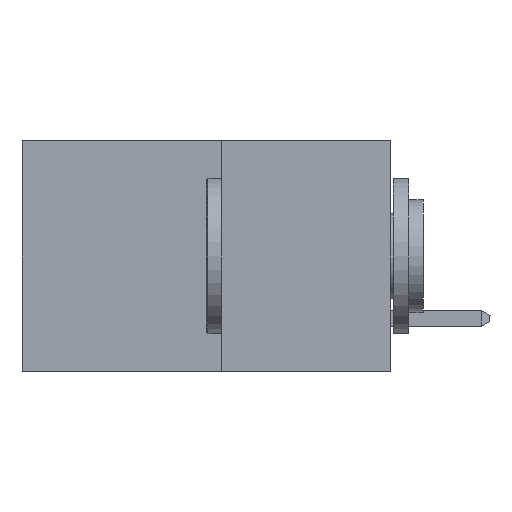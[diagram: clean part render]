
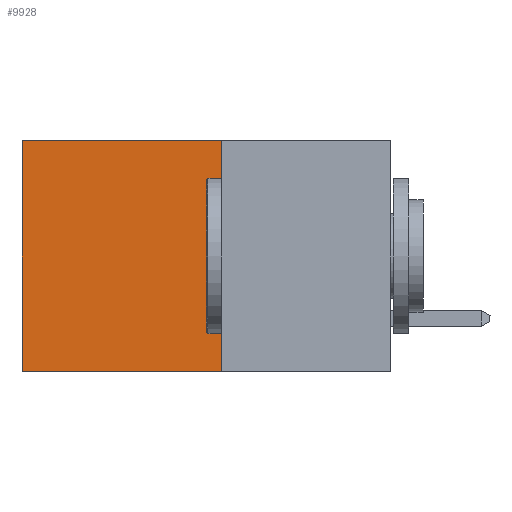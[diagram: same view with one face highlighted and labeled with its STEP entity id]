
A CAD part, left-side view. The second image highlights one B-rep face of the part: STEP entity #9928.
In plain terms, the highlighted planar face has unit normal (-1, 0, 0).
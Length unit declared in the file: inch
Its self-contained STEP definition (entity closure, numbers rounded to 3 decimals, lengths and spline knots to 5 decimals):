
#417 = DIRECTION ( 'NONE',  ( 0., 0., -1. ) ) ;
#490 = VECTOR ( 'NONE', #26340, 39.37008 ) ;
#1236 = ORIENTED_EDGE ( 'NONE', *, *, #13361, .F. ) ;
#3910 = CARTESIAN_POINT ( 'NONE',  ( 0.277, 0.59, 0. ) ) ;
#5032 = CARTESIAN_POINT ( 'NONE',  ( 0.277, 0.27, 0. ) ) ;
#5925 = LINE ( 'NONE', #8817, #16747 ) ;
#6266 = VERTEX_POINT ( 'NONE', #3910 ) ;
#6485 = VECTOR ( 'NONE', #9654, 39.37008 ) ;
#8775 = ORIENTED_EDGE ( 'NONE', *, *, #8777, .F. ) ;
#8777 = EDGE_CURVE ( 'NONE', #9025, #25424, #19285, .T. ) ;
#8817 = CARTESIAN_POINT ( 'NONE',  ( 0.277, 0.27, -0.37 ) ) ;
#9025 = VERTEX_POINT ( 'NONE', #25426 ) ;
#9540 = VERTEX_POINT ( 'NONE', #16863 ) ;
#9654 = DIRECTION ( 'NONE',  ( 0., 0., -1. ) ) ;
#9928 = ADVANCED_FACE ( 'NONE', ( #11229 ), #24043, .F. ) ;
#9935 = ORIENTED_EDGE ( 'NONE', *, *, #23583, .T. ) ;
#11036 = DIRECTION ( 'NONE',  ( 0., 1., 0. ) ) ;
#11229 = FACE_OUTER_BOUND ( 'NONE', #14681, .T. ) ;
#11257 = CARTESIAN_POINT ( 'NONE',  ( 0.277, 0.27, -0.37 ) ) ;
#11324 = EDGE_CURVE ( 'NONE', #6266, #9540, #26089, .T. ) ;
#11795 = CARTESIAN_POINT ( 'NONE',  ( 0.277, 0.27, -0.37 ) ) ;
#13361 = EDGE_CURVE ( 'NONE', #25424, #9540, #5925, .T. ) ;
#13459 = DIRECTION ( 'NONE',  ( 1., 0., 0. ) ) ;
#13855 = CARTESIAN_POINT ( 'NONE',  ( 0.277, 0.59, -0.37 ) ) ;
#14681 = EDGE_LOOP ( 'NONE', ( #19759, #1236, #8775, #9935 ) ) ;
#15970 = DIRECTION ( 'NONE',  ( 0., 0., -1. ) ) ;
#16747 = VECTOR ( 'NONE', #11036, 39.37008 ) ;
#16863 = CARTESIAN_POINT ( 'NONE',  ( 0.277, 0.59, -0.37 ) ) ;
#17655 = AXIS2_PLACEMENT_3D ( 'NONE', #11257, #13459, #417 ) ;
#18344 = LINE ( 'NONE', #5032, #490 ) ;
#19285 = LINE ( 'NONE', #11795, #6485 ) ;
#19759 = ORIENTED_EDGE ( 'NONE', *, *, #11324, .T. ) ;
#20467 = CARTESIAN_POINT ( 'NONE',  ( 0.277, 0.27, -0.37 ) ) ;
#20500 = VECTOR ( 'NONE', #15970, 39.37008 ) ;
#23583 = EDGE_CURVE ( 'NONE', #9025, #6266, #18344, .T. ) ;
#24043 = PLANE ( 'NONE',  #17655 ) ;
#25424 = VERTEX_POINT ( 'NONE', #20467 ) ;
#25426 = CARTESIAN_POINT ( 'NONE',  ( 0.277, 0.27, 0. ) ) ;
#26089 = LINE ( 'NONE', #13855, #20500 ) ;
#26340 = DIRECTION ( 'NONE',  ( 0., 1., 0. ) ) ;
